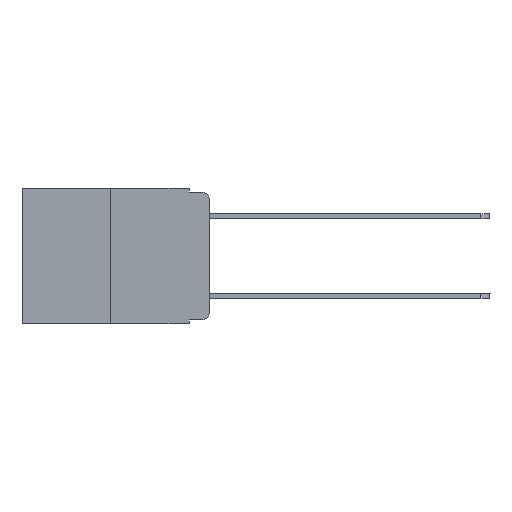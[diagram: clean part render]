
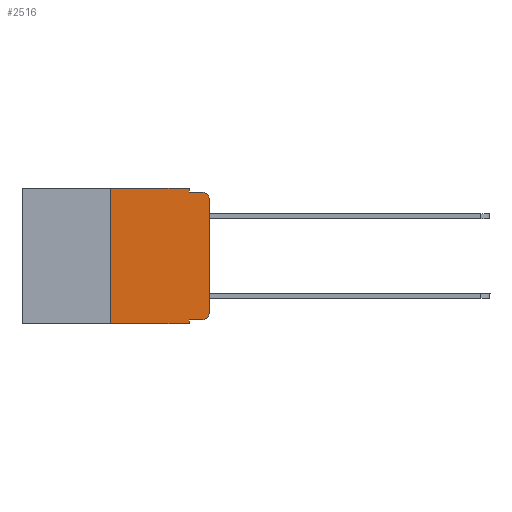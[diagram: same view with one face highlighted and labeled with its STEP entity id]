
A CAD part, left-side view. The second image highlights one B-rep face of the part: STEP entity #2516.
In plain terms, the highlighted planar face has unit normal (-1, 0, 0).
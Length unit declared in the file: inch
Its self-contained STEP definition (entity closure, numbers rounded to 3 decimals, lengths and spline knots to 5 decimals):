
#111 = VECTOR ( 'NONE', #13340, 39.37008 ) ;
#201 = ORIENTED_EDGE ( 'NONE', *, *, #2081, .F. ) ;
#578 = VERTEX_POINT ( 'NONE', #6857 ) ;
#938 = VERTEX_POINT ( 'NONE', #3519 ) ;
#1062 = ORIENTED_EDGE ( 'NONE', *, *, #6579, .T. ) ;
#1435 = VERTEX_POINT ( 'NONE', #12221 ) ;
#1561 = VERTEX_POINT ( 'NONE', #6039 ) ;
#1637 = EDGE_CURVE ( 'NONE', #13375, #5526, #4902, .T. ) ;
#1724 = VECTOR ( 'NONE', #2725, 39.37008 ) ;
#1801 = AXIS2_PLACEMENT_3D ( 'NONE', #1907, #9335, #12749 ) ;
#1813 = CARTESIAN_POINT ( 'NONE',  ( 0., 0.473, 0. ) ) ;
#1890 = PLANE ( 'NONE',  #10204 ) ;
#1907 = CARTESIAN_POINT ( 'NONE',  ( 0., 0.02, -0.03 ) ) ;
#2081 = EDGE_CURVE ( 'NONE', #1561, #7062, #3889, .T. ) ;
#2334 = LINE ( 'NONE', #3524, #3200 ) ;
#2516 = ADVANCED_FACE ( 'NONE', ( #4924 ), #1890, .F. ) ;
#2562 = CARTESIAN_POINT ( 'NONE',  ( 0., 0.25, -0.343 ) ) ;
#2647 = CARTESIAN_POINT ( 'NONE',  ( 0., 0.02, -0.313 ) ) ;
#2725 = DIRECTION ( 'NONE',  ( 0., -1., 0. ) ) ;
#2738 = CARTESIAN_POINT ( 'NONE',  ( 0., 0.473, -0.343 ) ) ;
#3126 = CARTESIAN_POINT ( 'NONE',  ( 0., 0.051, -0.343 ) ) ;
#3129 = LINE ( 'NONE', #7446, #12582 ) ;
#3160 = ORIENTED_EDGE ( 'NONE', *, *, #1637, .T. ) ;
#3200 = VECTOR ( 'NONE', #7838, 39.37008 ) ;
#3331 = EDGE_CURVE ( 'NONE', #1435, #12437, #13235, .T. ) ;
#3394 = EDGE_CURVE ( 'NONE', #7062, #578, #9145, .T. ) ;
#3519 = CARTESIAN_POINT ( 'NONE',  ( 0., 0., -0.03 ) ) ;
#3524 = CARTESIAN_POINT ( 'NONE',  ( 0., 0.051, 0. ) ) ;
#3615 = CIRCLE ( 'NONE', #1801, 0.02 ) ;
#3694 = VECTOR ( 'NONE', #12504, 39.37008 ) ;
#3889 = LINE ( 'NONE', #9555, #9542 ) ;
#4825 = DIRECTION ( 'NONE',  ( 0., 0., -1. ) ) ;
#4902 = LINE ( 'NONE', #2738, #3694 ) ;
#4924 = FACE_OUTER_BOUND ( 'NONE', #11973, .T. ) ;
#5125 = EDGE_CURVE ( 'NONE', #578, #10163, #7018, .T. ) ;
#5198 = VECTOR ( 'NONE', #4825, 39.37008 ) ;
#5526 = VERTEX_POINT ( 'NONE', #3126 ) ;
#5605 = EDGE_CURVE ( 'NONE', #12437, #938, #12401, .T. ) ;
#5694 = ORIENTED_EDGE ( 'NONE', *, *, #11691, .T. ) ;
#6039 = CARTESIAN_POINT ( 'NONE',  ( 0., 0.25, 0. ) ) ;
#6579 = EDGE_CURVE ( 'NONE', #11850, #1435, #3129, .T. ) ;
#6857 = CARTESIAN_POINT ( 'NONE',  ( 0., 0.051, -0.01 ) ) ;
#6943 = DIRECTION ( 'NONE',  ( 0., 0., -1. ) ) ;
#7018 = LINE ( 'NONE', #10096, #1724 ) ;
#7062 = VERTEX_POINT ( 'NONE', #11638 ) ;
#7446 = CARTESIAN_POINT ( 'NONE',  ( 0., 0.051, -0.333 ) ) ;
#7783 = AXIS2_PLACEMENT_3D ( 'NONE', #2647, #11147, #6943 ) ;
#7838 = DIRECTION ( 'NONE',  ( 0., 0., -1. ) ) ;
#7906 = ORIENTED_EDGE ( 'NONE', *, *, #11618, .F. ) ;
#8079 = CARTESIAN_POINT ( 'NONE',  ( 0., 0.051, 0. ) ) ;
#8555 = CARTESIAN_POINT ( 'NONE',  ( 0., 0.051, -0.333 ) ) ;
#9007 = ORIENTED_EDGE ( 'NONE', *, *, #5125, .F. ) ;
#9145 = LINE ( 'NONE', #8079, #5198 ) ;
#9335 = DIRECTION ( 'NONE',  ( -1., 0., 0. ) ) ;
#9542 = VECTOR ( 'NONE', #12539, 39.37008 ) ;
#9555 = CARTESIAN_POINT ( 'NONE',  ( 0., 0.473, 0. ) ) ;
#9614 = ORIENTED_EDGE ( 'NONE', *, *, #5605, .T. ) ;
#9928 = CARTESIAN_POINT ( 'NONE',  ( 0., 0.25, 0. ) ) ;
#10073 = LINE ( 'NONE', #9928, #13798 ) ;
#10096 = CARTESIAN_POINT ( 'NONE',  ( 0., 0.051, -0.01 ) ) ;
#10163 = VERTEX_POINT ( 'NONE', #11716 ) ;
#10204 = AXIS2_PLACEMENT_3D ( 'NONE', #1813, #11681, #12526 ) ;
#11147 = DIRECTION ( 'NONE',  ( -1., 0., 0. ) ) ;
#11216 = CARTESIAN_POINT ( 'NONE',  ( 0., 0., -0.313 ) ) ;
#11311 = DIRECTION ( 'NONE',  ( 0., -1., 0. ) ) ;
#11344 = CARTESIAN_POINT ( 'NONE',  ( 0., 0., 0. ) ) ;
#11618 = EDGE_CURVE ( 'NONE', #13375, #1561, #10073, .T. ) ;
#11638 = CARTESIAN_POINT ( 'NONE',  ( 0., 0.051, 0. ) ) ;
#11681 = DIRECTION ( 'NONE',  ( 1., 0., 0. ) ) ;
#11691 = EDGE_CURVE ( 'NONE', #938, #10163, #3615, .T. ) ;
#11716 = CARTESIAN_POINT ( 'NONE',  ( 0., 0.02, -0.01 ) ) ;
#11815 = ORIENTED_EDGE ( 'NONE', *, *, #3394, .F. ) ;
#11850 = VERTEX_POINT ( 'NONE', #8555 ) ;
#11973 = EDGE_LOOP ( 'NONE', ( #9614, #5694, #9007, #11815, #201, #7906, #3160, #13860, #1062, #13803 ) ) ;
#12121 = DIRECTION ( 'NONE',  ( 0., 0., 1. ) ) ;
#12221 = CARTESIAN_POINT ( 'NONE',  ( 0., 0.02, -0.333 ) ) ;
#12401 = LINE ( 'NONE', #11344, #111 ) ;
#12437 = VERTEX_POINT ( 'NONE', #11216 ) ;
#12504 = DIRECTION ( 'NONE',  ( 0., -1., 0. ) ) ;
#12526 = DIRECTION ( 'NONE',  ( 0., 0., -1. ) ) ;
#12539 = DIRECTION ( 'NONE',  ( 0., -1., 0. ) ) ;
#12582 = VECTOR ( 'NONE', #11311, 39.37008 ) ;
#12749 = DIRECTION ( 'NONE',  ( 0., 0., -1. ) ) ;
#13235 = CIRCLE ( 'NONE', #7783, 0.02 ) ;
#13340 = DIRECTION ( 'NONE',  ( 0., 0., 1. ) ) ;
#13375 = VERTEX_POINT ( 'NONE', #2562 ) ;
#13790 = EDGE_CURVE ( 'NONE', #11850, #5526, #2334, .T. ) ;
#13798 = VECTOR ( 'NONE', #12121, 39.37008 ) ;
#13803 = ORIENTED_EDGE ( 'NONE', *, *, #3331, .T. ) ;
#13860 = ORIENTED_EDGE ( 'NONE', *, *, #13790, .F. ) ;
